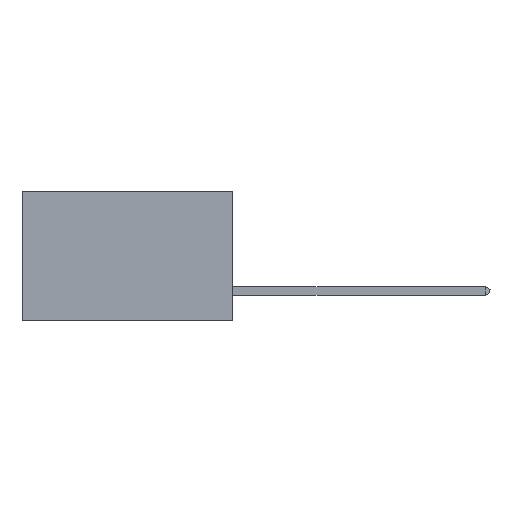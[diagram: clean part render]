
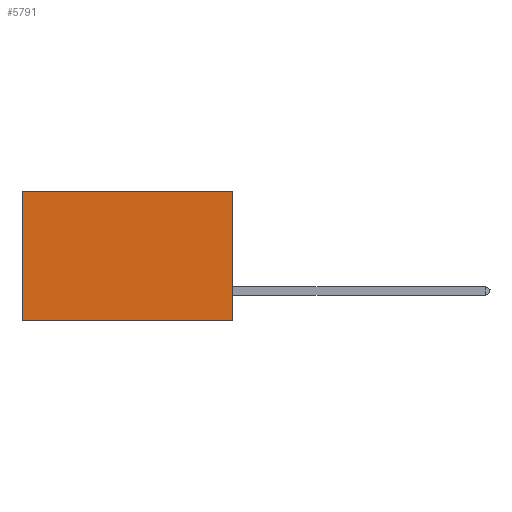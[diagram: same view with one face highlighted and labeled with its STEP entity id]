
A CAD part, left-side view. The second image highlights one B-rep face of the part: STEP entity #5791.
In plain terms, the highlighted planar face has unit normal (-1, 0, 0).
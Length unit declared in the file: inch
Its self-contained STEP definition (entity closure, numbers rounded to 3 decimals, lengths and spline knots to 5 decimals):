
#373 = VECTOR ( 'NONE', #41207, 39.37008 ) ;
#1993 = EDGE_LOOP ( 'NONE', ( #29734, #32364, #29664, #29833 ) ) ;
#2476 = CARTESIAN_POINT ( 'NONE',  ( 0.2875, 0., 0. ) ) ;
#5011 = DIRECTION ( 'NONE',  ( 0., 1., 0. ) ) ;
#5135 = EDGE_CURVE ( 'NONE', #6710, #35662, #29627, .T. ) ;
#5791 = ADVANCED_FACE ( 'NONE', ( #35719 ), #38207, .F. ) ;
#6710 = VERTEX_POINT ( 'NONE', #30260 ) ;
#8893 = EDGE_CURVE ( 'NONE', #18333, #11795, #31377, .T. ) ;
#8909 = DIRECTION ( 'NONE',  ( 0., 0., -1. ) ) ;
#10970 = AXIS2_PLACEMENT_3D ( 'NONE', #2476, #15120, #8909 ) ;
#11795 = VERTEX_POINT ( 'NONE', #12184 ) ;
#12184 = CARTESIAN_POINT ( 'NONE',  ( 0.2875, 0.6, -0.37 ) ) ;
#13877 = VECTOR ( 'NONE', #27454, 39.37008 ) ;
#14681 = LINE ( 'NONE', #28336, #373 ) ;
#15120 = DIRECTION ( 'NONE',  ( 1., 0., 0. ) ) ;
#15991 = VECTOR ( 'NONE', #26900, 39.37008 ) ;
#18333 = VERTEX_POINT ( 'NONE', #34796 ) ;
#19556 = EDGE_CURVE ( 'NONE', #35662, #11795, #14681, .T. ) ;
#23163 = LINE ( 'NONE', #39651, #15991 ) ;
#26900 = DIRECTION ( 'NONE',  ( 0., 0., -1. ) ) ;
#27454 = DIRECTION ( 'NONE',  ( 0., 1., 0. ) ) ;
#27798 = EDGE_CURVE ( 'NONE', #6710, #18333, #23163, .T. ) ;
#28336 = CARTESIAN_POINT ( 'NONE',  ( 0.2875, 0.6, 0. ) ) ;
#28954 = CARTESIAN_POINT ( 'NONE',  ( 0.2875, 0.6, 0. ) ) ;
#29627 = LINE ( 'NONE', #34595, #32181 ) ;
#29664 = ORIENTED_EDGE ( 'NONE', *, *, #27798, .F. ) ;
#29734 = ORIENTED_EDGE ( 'NONE', *, *, #19556, .T. ) ;
#29833 = ORIENTED_EDGE ( 'NONE', *, *, #5135, .T. ) ;
#30260 = CARTESIAN_POINT ( 'NONE',  ( 0.2875, 0., 0. ) ) ;
#31377 = LINE ( 'NONE', #34453, #13877 ) ;
#32181 = VECTOR ( 'NONE', #5011, 39.37008 ) ;
#32364 = ORIENTED_EDGE ( 'NONE', *, *, #8893, .F. ) ;
#34453 = CARTESIAN_POINT ( 'NONE',  ( 0.2875, 0., -0.37 ) ) ;
#34595 = CARTESIAN_POINT ( 'NONE',  ( 0.2875, 0., 0. ) ) ;
#34796 = CARTESIAN_POINT ( 'NONE',  ( 0.2875, 0., -0.37 ) ) ;
#35662 = VERTEX_POINT ( 'NONE', #28954 ) ;
#35719 = FACE_OUTER_BOUND ( 'NONE', #1993, .T. ) ;
#38207 = PLANE ( 'NONE',  #10970 ) ;
#39651 = CARTESIAN_POINT ( 'NONE',  ( 0.2875, 0., 0. ) ) ;
#41207 = DIRECTION ( 'NONE',  ( 0., 0., -1. ) ) ;
